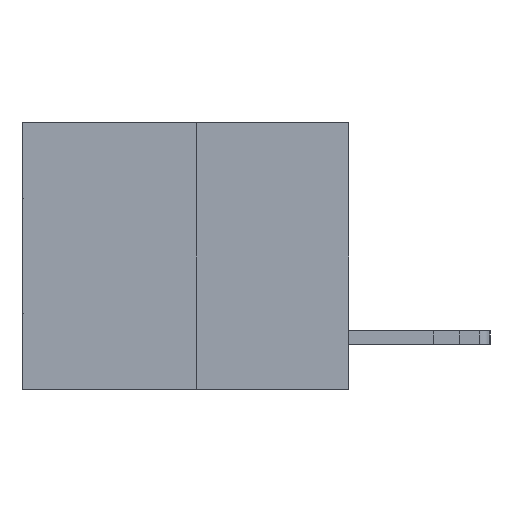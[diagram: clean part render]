
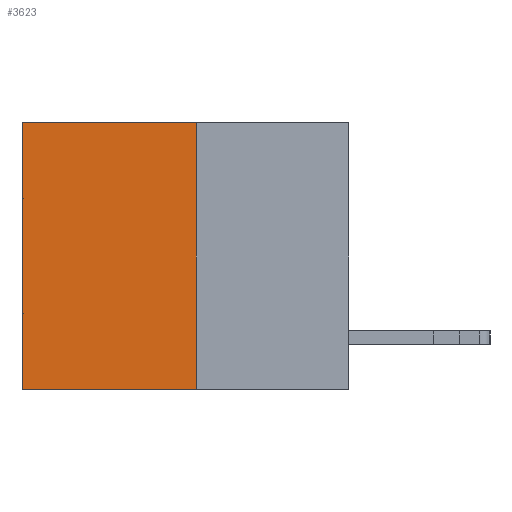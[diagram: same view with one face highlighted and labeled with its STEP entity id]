
A CAD part, left-side view. The second image highlights one B-rep face of the part: STEP entity #3623.
In plain terms, the highlighted planar face has unit normal (-1, 0, 0).
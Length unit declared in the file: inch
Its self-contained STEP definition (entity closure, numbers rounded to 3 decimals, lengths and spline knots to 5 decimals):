
#577 = CARTESIAN_POINT ( 'NONE',  ( 0.3165, 0.28, 0. ) ) ;
#807 = DIRECTION ( 'NONE',  ( 0., 0., -1. ) ) ;
#1435 = VECTOR ( 'NONE', #807, 39.37008 ) ;
#1585 = ORIENTED_EDGE ( 'NONE', *, *, #5973, .F. ) ;
#1613 = VERTEX_POINT ( 'NONE', #2453 ) ;
#1730 = DIRECTION ( 'NONE',  ( 0., 0., -1. ) ) ;
#1910 = LINE ( 'NONE', #13521, #8628 ) ;
#2373 = EDGE_CURVE ( 'NONE', #17282, #27413, #5522, .T. ) ;
#2453 = CARTESIAN_POINT ( 'NONE',  ( 0.3165, 0.28, -0.49 ) ) ;
#3041 = VERTEX_POINT ( 'NONE', #577 ) ;
#3623 = ADVANCED_FACE ( 'NONE', ( #28583 ), #22668, .F. ) ;
#3703 = DIRECTION ( 'NONE',  ( 0., 1., 0. ) ) ;
#5299 = CARTESIAN_POINT ( 'NONE',  ( 0.3165, 0.6, -0.49 ) ) ;
#5522 = LINE ( 'NONE', #5299, #1435 ) ;
#5542 = CARTESIAN_POINT ( 'NONE',  ( 0.3165, 0.28, -0.49 ) ) ;
#5834 = LINE ( 'NONE', #8665, #8453 ) ;
#5973 = EDGE_CURVE ( 'NONE', #3041, #1613, #1910, .T. ) ;
#6524 = CARTESIAN_POINT ( 'NONE',  ( 0.3165, 0.6, -0.49 ) ) ;
#6666 = EDGE_CURVE ( 'NONE', #1613, #27413, #22472, .T. ) ;
#8453 = VECTOR ( 'NONE', #3703, 39.37008 ) ;
#8628 = VECTOR ( 'NONE', #1730, 39.37008 ) ;
#8665 = CARTESIAN_POINT ( 'NONE',  ( 0.3165, 0.28, 0. ) ) ;
#11920 = CARTESIAN_POINT ( 'NONE',  ( 0.3165, 0.6, 0. ) ) ;
#12083 = CARTESIAN_POINT ( 'NONE',  ( 0.3165, 0.28, -0.49 ) ) ;
#13223 = EDGE_CURVE ( 'NONE', #3041, #17282, #5834, .T. ) ;
#13521 = CARTESIAN_POINT ( 'NONE',  ( 0.3165, 0.28, -0.49 ) ) ;
#15690 = DIRECTION ( 'NONE',  ( 0., 0., -1. ) ) ;
#17282 = VERTEX_POINT ( 'NONE', #11920 ) ;
#18957 = ORIENTED_EDGE ( 'NONE', *, *, #13223, .T. ) ;
#19954 = DIRECTION ( 'NONE',  ( 1., 0., 0. ) ) ;
#20189 = VECTOR ( 'NONE', #28798, 39.37008 ) ;
#20899 = ORIENTED_EDGE ( 'NONE', *, *, #2373, .T. ) ;
#20945 = ORIENTED_EDGE ( 'NONE', *, *, #6666, .F. ) ;
#22448 = EDGE_LOOP ( 'NONE', ( #20899, #20945, #1585, #18957 ) ) ;
#22472 = LINE ( 'NONE', #12083, #20189 ) ;
#22668 = PLANE ( 'NONE',  #23137 ) ;
#23137 = AXIS2_PLACEMENT_3D ( 'NONE', #5542, #19954, #15690 ) ;
#27413 = VERTEX_POINT ( 'NONE', #6524 ) ;
#28583 = FACE_OUTER_BOUND ( 'NONE', #22448, .T. ) ;
#28798 = DIRECTION ( 'NONE',  ( 0., 1., 0. ) ) ;
